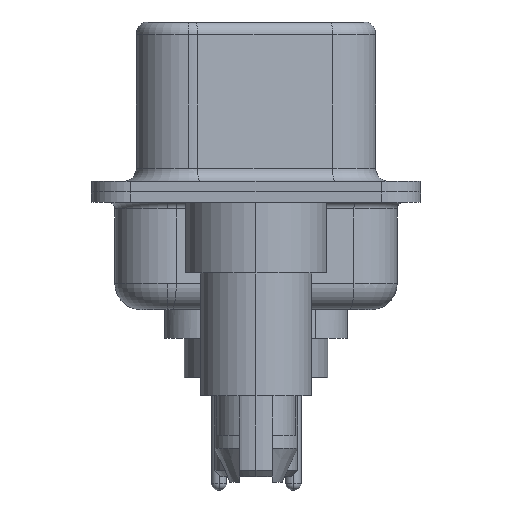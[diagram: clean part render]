
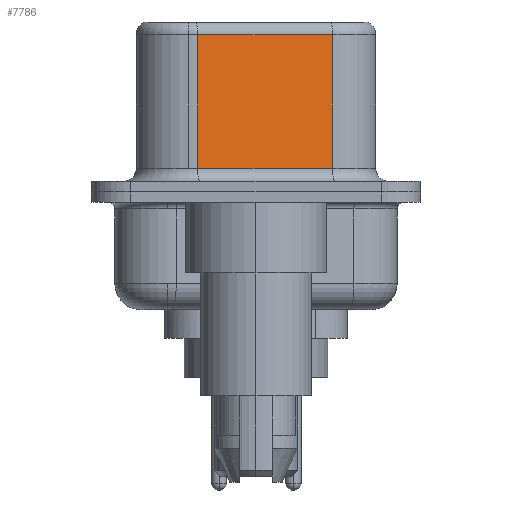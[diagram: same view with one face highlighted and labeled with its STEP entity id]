
A CAD part, left-side view. The second image highlights one B-rep face of the part: STEP entity #7786.
In plain terms, the highlighted planar face has unit normal (-0.985, -0.174, 0).
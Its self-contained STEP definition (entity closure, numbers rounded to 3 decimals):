
#515 = ORIENTED_EDGE ( 'NONE', *, *, #4175, .T. ) ;
#548 = VECTOR ( 'NONE', #841, 1000. ) ;
#841 = DIRECTION ( 'NONE',  ( -0.174, 0.985, 0. ) ) ;
#1241 = DIRECTION ( 'NONE',  ( 0.174, -0.985, 0. ) ) ;
#1410 = DIRECTION ( 'NONE',  ( 0., 0., -1. ) ) ;
#3262 = ORIENTED_EDGE ( 'NONE', *, *, #16300, .F. ) ;
#4175 = EDGE_CURVE ( 'NONE', #8016, #16670, #17894, .T. ) ;
#4260 = ORIENTED_EDGE ( 'NONE', *, *, #11381, .T. ) ;
#5189 = DIRECTION ( 'NONE',  ( 0., 0., -1. ) ) ;
#6681 = EDGE_LOOP ( 'NONE', ( #3262, #8037, #4260, #515 ) ) ;
#7685 = VECTOR ( 'NONE', #5189, 1000. ) ;
#7786 = ADVANCED_FACE ( 'NONE', ( #18804 ), #18732, .F. ) ;
#8016 = VERTEX_POINT ( 'NONE', #13655 ) ;
#8037 = ORIENTED_EDGE ( 'NONE', *, *, #9781, .T. ) ;
#8770 = CARTESIAN_POINT ( 'NONE',  ( 4.565, -2.927, 0.9 ) ) ;
#9781 = EDGE_CURVE ( 'NONE', #13609, #14669, #13783, .T. ) ;
#10998 = CARTESIAN_POINT ( 'NONE',  ( 4.565, -2.927, 6.52 ) ) ;
#11381 = EDGE_CURVE ( 'NONE', #14669, #8016, #19382, .T. ) ;
#11580 = CARTESIAN_POINT ( 'NONE',  ( 4.565, -2.927, 0.9 ) ) ;
#12844 = CARTESIAN_POINT ( 'NONE',  ( 3.655, 2.233, 6.02 ) ) ;
#13609 = VERTEX_POINT ( 'NONE', #14406 ) ;
#13655 = CARTESIAN_POINT ( 'NONE',  ( 3.655, 2.233, 0.9 ) ) ;
#13722 = VECTOR ( 'NONE', #1241, 1000. ) ;
#13783 = LINE ( 'NONE', #19959, #548 ) ;
#13931 = AXIS2_PLACEMENT_3D ( 'NONE', #19734, #18417, #18397 ) ;
#14406 = CARTESIAN_POINT ( 'NONE',  ( 4.565, -2.927, 6.02 ) ) ;
#14669 = VERTEX_POINT ( 'NONE', #12844 ) ;
#16300 = EDGE_CURVE ( 'NONE', #13609, #16670, #18691, .T. ) ;
#16313 = CARTESIAN_POINT ( 'NONE',  ( 3.655, 2.233, 6.52 ) ) ;
#16670 = VERTEX_POINT ( 'NONE', #8770 ) ;
#17894 = LINE ( 'NONE', #11580, #13722 ) ;
#18397 = DIRECTION ( 'NONE',  ( -0.174, 0.985, 0. ) ) ;
#18417 = DIRECTION ( 'NONE',  ( 0.985, 0.174, 0. ) ) ;
#18691 = LINE ( 'NONE', #10998, #19733 ) ;
#18732 = PLANE ( 'NONE',  #13931 ) ;
#18804 = FACE_OUTER_BOUND ( 'NONE', #6681, .T. ) ;
#19382 = LINE ( 'NONE', #16313, #7685 ) ;
#19733 = VECTOR ( 'NONE', #1410, 1000. ) ;
#19734 = CARTESIAN_POINT ( 'NONE',  ( 4.565, -2.927, 6.52 ) ) ;
#19959 = CARTESIAN_POINT ( 'NONE',  ( 4.565, -2.927, 6.02 ) ) ;
